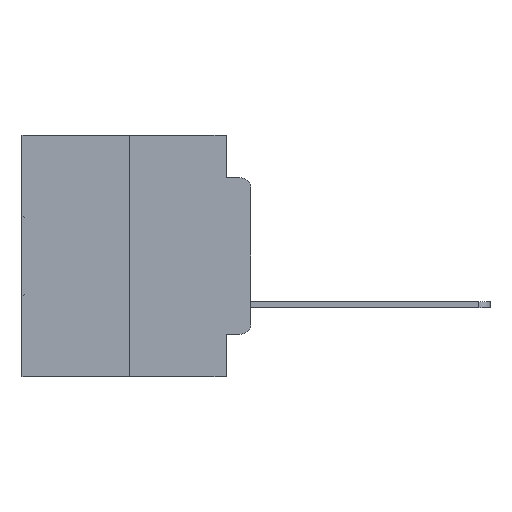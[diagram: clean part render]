
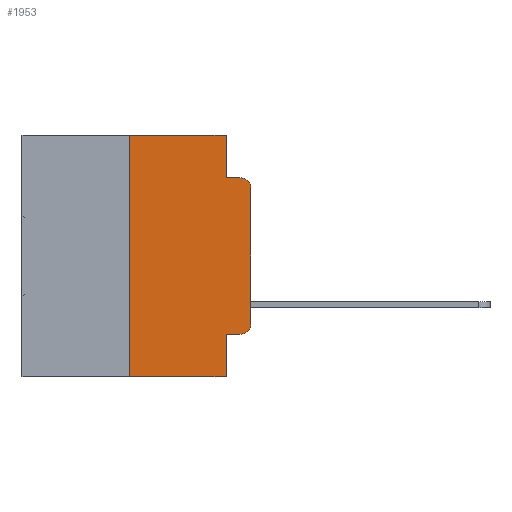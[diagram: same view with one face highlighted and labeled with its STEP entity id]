
A CAD part, left-side view. The second image highlights one B-rep face of the part: STEP entity #1953.
In plain terms, the highlighted planar face has unit normal (-1, 0, 0).
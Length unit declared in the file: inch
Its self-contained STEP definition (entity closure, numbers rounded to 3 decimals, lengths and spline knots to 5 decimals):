
#313 = EDGE_CURVE ( 'NONE', #1375, #4841, #18446, .T. ) ;
#980 = VECTOR ( 'NONE', #13861, 39.37008 ) ;
#1031 = EDGE_CURVE ( 'NONE', #4841, #5016, #9998, .T. ) ;
#1154 = AXIS2_PLACEMENT_3D ( 'NONE', #28250, #14088, #30470 ) ;
#1375 = VERTEX_POINT ( 'NONE', #27330 ) ;
#1814 = LINE ( 'NONE', #30266, #980 ) ;
#1822 = ORIENTED_EDGE ( 'NONE', *, *, #5823, .T. ) ;
#1953 = ADVANCED_FACE ( 'NONE', ( #25791 ), #24351, .F. ) ;
#2005 = LINE ( 'NONE', #16626, #16105 ) ;
#2744 = CARTESIAN_POINT ( 'NONE',  ( 0., 0.25, 0. ) ) ;
#3236 = VERTEX_POINT ( 'NONE', #20548 ) ;
#3246 = EDGE_CURVE ( 'NONE', #5016, #4764, #30574, .T. ) ;
#3471 = ORIENTED_EDGE ( 'NONE', *, *, #21327, .T. ) ;
#3525 = DIRECTION ( 'NONE',  ( 0., -1., 0. ) ) ;
#3994 = CARTESIAN_POINT ( 'NONE',  ( 0., 0., -0.1085 ) ) ;
#4331 = AXIS2_PLACEMENT_3D ( 'NONE', #5236, #22424, #7826 ) ;
#4624 = LINE ( 'NONE', #25945, #29495 ) ;
#4688 = ORIENTED_EDGE ( 'NONE', *, *, #9181, .T. ) ;
#4712 = CARTESIAN_POINT ( 'NONE',  ( 0., 0.473, 0. ) ) ;
#4764 = VERTEX_POINT ( 'NONE', #12553 ) ;
#4841 = VERTEX_POINT ( 'NONE', #2744 ) ;
#5016 = VERTEX_POINT ( 'NONE', #23058 ) ;
#5236 = CARTESIAN_POINT ( 'NONE',  ( 0., 0.02, -0.1085 ) ) ;
#5432 = CARTESIAN_POINT ( 'NONE',  ( 0., 0.051, -0.4115 ) ) ;
#5642 = VERTEX_POINT ( 'NONE', #18260 ) ;
#5823 = EDGE_CURVE ( 'NONE', #1375, #13806, #2005, .T. ) ;
#6168 = EDGE_LOOP ( 'NONE', ( #4688, #17839, #12888, #25668, #7939, #20923, #1822, #22440, #3471, #23924 ) ) ;
#6992 = EDGE_CURVE ( 'NONE', #4764, #14895, #14161, .T. ) ;
#7416 = EDGE_CURVE ( 'NONE', #19112, #14895, #22089, .T. ) ;
#7627 = VECTOR ( 'NONE', #3525, 39.37008 ) ;
#7826 = DIRECTION ( 'NONE',  ( 0., 0., -1. ) ) ;
#7939 = ORIENTED_EDGE ( 'NONE', *, *, #1031, .F. ) ;
#8328 = VECTOR ( 'NONE', #15598, 39.37008 ) ;
#9181 = EDGE_CURVE ( 'NONE', #3236, #19112, #4624, .T. ) ;
#9387 = CARTESIAN_POINT ( 'NONE',  ( 0., 0.02, -0.0885 ) ) ;
#9810 = DIRECTION ( 'NONE',  ( 1., 0., 0. ) ) ;
#9998 = LINE ( 'NONE', #20827, #16460 ) ;
#10769 = VECTOR ( 'NONE', #15113, 39.37008 ) ;
#11250 = CARTESIAN_POINT ( 'NONE',  ( 0., 0.25, 0. ) ) ;
#11944 = VECTOR ( 'NONE', #28400, 39.37008 ) ;
#12553 = CARTESIAN_POINT ( 'NONE',  ( 0., 0.051, -0.0885 ) ) ;
#12888 = ORIENTED_EDGE ( 'NONE', *, *, #6992, .F. ) ;
#13525 = CARTESIAN_POINT ( 'NONE',  ( 0., 0.051, -0.0885 ) ) ;
#13806 = VERTEX_POINT ( 'NONE', #14666 ) ;
#13861 = DIRECTION ( 'NONE',  ( 0., -1., 0. ) ) ;
#13937 = DIRECTION ( 'NONE',  ( 0., 0., 1. ) ) ;
#13983 = VERTEX_POINT ( 'NONE', #5432 ) ;
#14088 = DIRECTION ( 'NONE',  ( -1., 0., 0. ) ) ;
#14161 = LINE ( 'NONE', #13525, #7627 ) ;
#14246 = EDGE_CURVE ( 'NONE', #5642, #3236, #17240, .T. ) ;
#14666 = CARTESIAN_POINT ( 'NONE',  ( 0., 0.051, -0.5 ) ) ;
#14895 = VERTEX_POINT ( 'NONE', #9387 ) ;
#15113 = DIRECTION ( 'NONE',  ( 0., 0., -1. ) ) ;
#15598 = DIRECTION ( 'NONE',  ( 0., 0., -1. ) ) ;
#16105 = VECTOR ( 'NONE', #30597, 39.37008 ) ;
#16460 = VECTOR ( 'NONE', #20920, 39.37008 ) ;
#16626 = CARTESIAN_POINT ( 'NONE',  ( 0., 0.473, -0.5 ) ) ;
#17240 = CIRCLE ( 'NONE', #1154, 0.02 ) ;
#17839 = ORIENTED_EDGE ( 'NONE', *, *, #7416, .T. ) ;
#18125 = AXIS2_PLACEMENT_3D ( 'NONE', #4712, #9810, #26595 ) ;
#18260 = CARTESIAN_POINT ( 'NONE',  ( 0., 0.02, -0.4115 ) ) ;
#18446 = LINE ( 'NONE', #11250, #11944 ) ;
#19112 = VERTEX_POINT ( 'NONE', #3994 ) ;
#20548 = CARTESIAN_POINT ( 'NONE',  ( 0., 0., -0.3915 ) ) ;
#20827 = CARTESIAN_POINT ( 'NONE',  ( 0., 0.473, 0. ) ) ;
#20920 = DIRECTION ( 'NONE',  ( 0., -1., 0. ) ) ;
#20923 = ORIENTED_EDGE ( 'NONE', *, *, #313, .F. ) ;
#21327 = EDGE_CURVE ( 'NONE', #13983, #5642, #1814, .T. ) ;
#22089 = CIRCLE ( 'NONE', #4331, 0.02 ) ;
#22424 = DIRECTION ( 'NONE',  ( -1., 0., 0. ) ) ;
#22440 = ORIENTED_EDGE ( 'NONE', *, *, #24150, .F. ) ;
#23058 = CARTESIAN_POINT ( 'NONE',  ( 0., 0.051, 0. ) ) ;
#23924 = ORIENTED_EDGE ( 'NONE', *, *, #14246, .T. ) ;
#24150 = EDGE_CURVE ( 'NONE', #13983, #13806, #29707, .T. ) ;
#24351 = PLANE ( 'NONE',  #18125 ) ;
#25668 = ORIENTED_EDGE ( 'NONE', *, *, #3246, .F. ) ;
#25791 = FACE_OUTER_BOUND ( 'NONE', #6168, .T. ) ;
#25945 = CARTESIAN_POINT ( 'NONE',  ( 0., 0., 0. ) ) ;
#26595 = DIRECTION ( 'NONE',  ( 0., 0., -1. ) ) ;
#27330 = CARTESIAN_POINT ( 'NONE',  ( 0., 0.25, -0.5 ) ) ;
#27503 = CARTESIAN_POINT ( 'NONE',  ( 0., 0.051, 0. ) ) ;
#28250 = CARTESIAN_POINT ( 'NONE',  ( 0., 0.02, -0.3915 ) ) ;
#28400 = DIRECTION ( 'NONE',  ( 0., 0., 1. ) ) ;
#29205 = CARTESIAN_POINT ( 'NONE',  ( 0., 0.051, 0. ) ) ;
#29495 = VECTOR ( 'NONE', #13937, 39.37008 ) ;
#29707 = LINE ( 'NONE', #29205, #10769 ) ;
#30266 = CARTESIAN_POINT ( 'NONE',  ( 0., 0.051, -0.4115 ) ) ;
#30470 = DIRECTION ( 'NONE',  ( 0., 0., -1. ) ) ;
#30574 = LINE ( 'NONE', #27503, #8328 ) ;
#30597 = DIRECTION ( 'NONE',  ( 0., -1., 0. ) ) ;
